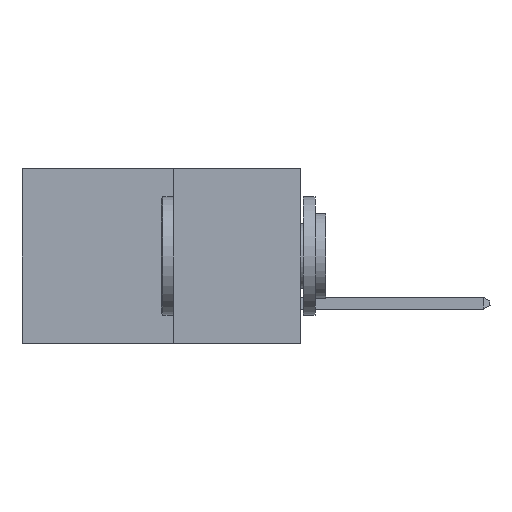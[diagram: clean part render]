
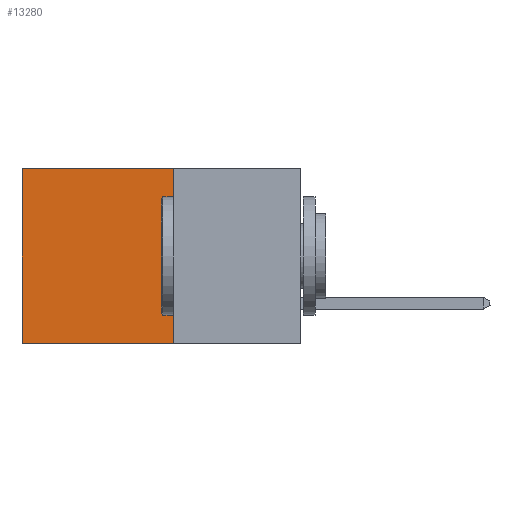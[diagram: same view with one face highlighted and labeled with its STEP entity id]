
A CAD part, left-side view. The second image highlights one B-rep face of the part: STEP entity #13280.
In plain terms, the highlighted planar face has unit normal (-1, 0, 0).
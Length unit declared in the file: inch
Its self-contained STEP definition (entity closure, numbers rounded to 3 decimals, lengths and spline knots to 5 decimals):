
#423 = ORIENTED_EDGE ( 'NONE', *, *, #1268, .F. ) ;
#658 = VERTEX_POINT ( 'NONE', #10668 ) ;
#1184 = CARTESIAN_POINT ( 'NONE',  ( 0.277, 0.27, 0. ) ) ;
#1268 = EDGE_CURVE ( 'NONE', #658, #2442, #4694, .T. ) ;
#1303 = ORIENTED_EDGE ( 'NONE', *, *, #2362, .F. ) ;
#1870 = VECTOR ( 'NONE', #12394, 39.37008 ) ;
#2153 = VECTOR ( 'NONE', #6394, 39.37008 ) ;
#2160 = DIRECTION ( 'NONE',  ( 0., 1., 0. ) ) ;
#2233 = CARTESIAN_POINT ( 'NONE',  ( 0.277, 0.27, -0.37 ) ) ;
#2326 = EDGE_LOOP ( 'NONE', ( #9981, #423, #1303, #3047 ) ) ;
#2357 = CARTESIAN_POINT ( 'NONE',  ( 0.277, 0.27, 0. ) ) ;
#2362 = EDGE_CURVE ( 'NONE', #13659, #658, #8751, .T. ) ;
#2442 = VERTEX_POINT ( 'NONE', #13310 ) ;
#3047 = ORIENTED_EDGE ( 'NONE', *, *, #4357, .T. ) ;
#3492 = DIRECTION ( 'NONE',  ( 0., 0., -1. ) ) ;
#3892 = CARTESIAN_POINT ( 'NONE',  ( 0.277, 0.59, -0.37 ) ) ;
#3906 = DIRECTION ( 'NONE',  ( 0., 0., -1. ) ) ;
#4357 = EDGE_CURVE ( 'NONE', #13659, #14231, #4716, .T. ) ;
#4470 = CARTESIAN_POINT ( 'NONE',  ( 0.277, 0.27, -0.37 ) ) ;
#4694 = LINE ( 'NONE', #4470, #1870 ) ;
#4716 = LINE ( 'NONE', #2357, #10782 ) ;
#5978 = VECTOR ( 'NONE', #3906, 39.37008 ) ;
#6031 = EDGE_CURVE ( 'NONE', #14231, #2442, #11928, .T. ) ;
#6394 = DIRECTION ( 'NONE',  ( 0., 0., -1. ) ) ;
#6769 = PLANE ( 'NONE',  #10367 ) ;
#7037 = CARTESIAN_POINT ( 'NONE',  ( 0.277, 0.59, 0. ) ) ;
#7955 = CARTESIAN_POINT ( 'NONE',  ( 0.277, 0.27, -0.37 ) ) ;
#8751 = LINE ( 'NONE', #7955, #2153 ) ;
#9981 = ORIENTED_EDGE ( 'NONE', *, *, #6031, .T. ) ;
#10350 = DIRECTION ( 'NONE',  ( 1., 0., 0. ) ) ;
#10367 = AXIS2_PLACEMENT_3D ( 'NONE', #2233, #10350, #3492 ) ;
#10668 = CARTESIAN_POINT ( 'NONE',  ( 0.277, 0.27, -0.37 ) ) ;
#10782 = VECTOR ( 'NONE', #2160, 39.37008 ) ;
#11928 = LINE ( 'NONE', #3892, #5978 ) ;
#12394 = DIRECTION ( 'NONE',  ( 0., 1., 0. ) ) ;
#13142 = FACE_OUTER_BOUND ( 'NONE', #2326, .T. ) ;
#13280 = ADVANCED_FACE ( 'NONE', ( #13142 ), #6769, .F. ) ;
#13310 = CARTESIAN_POINT ( 'NONE',  ( 0.277, 0.59, -0.37 ) ) ;
#13659 = VERTEX_POINT ( 'NONE', #1184 ) ;
#14231 = VERTEX_POINT ( 'NONE', #7037 ) ;
